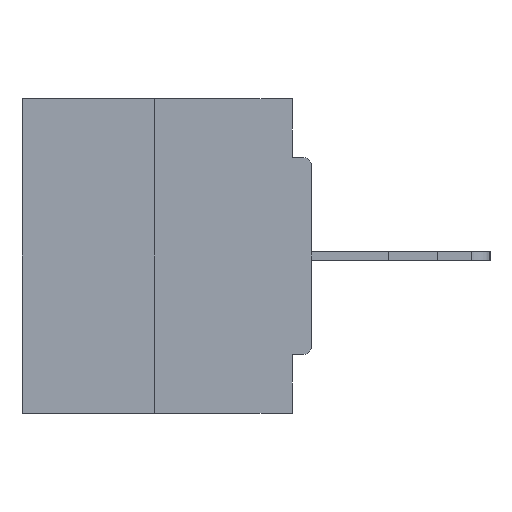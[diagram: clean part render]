
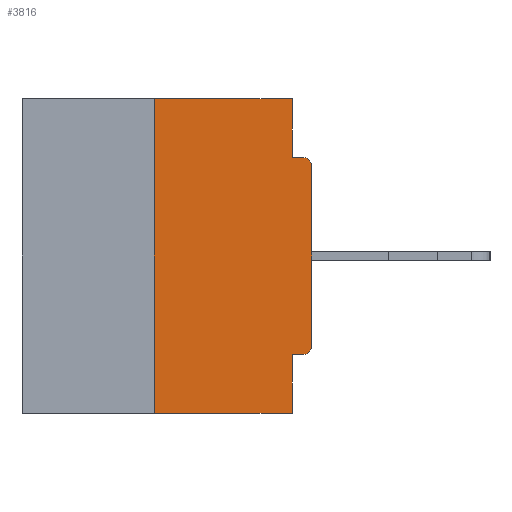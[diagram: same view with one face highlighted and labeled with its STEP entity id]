
A CAD part, left-side view. The second image highlights one B-rep face of the part: STEP entity #3816.
In plain terms, the highlighted planar face has unit normal (-1, 0, 0).
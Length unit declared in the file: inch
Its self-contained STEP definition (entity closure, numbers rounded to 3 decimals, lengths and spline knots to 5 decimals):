
#634 = CIRCLE ( 'NONE', #10946, 0.015 ) ;
#707 = CARTESIAN_POINT ( 'NONE',  ( 0., 0., -0.3915 ) ) ;
#1205 = VECTOR ( 'NONE', #3714, 39.37008 ) ;
#1463 = AXIS2_PLACEMENT_3D ( 'NONE', #26990, #29113, #23156 ) ;
#1750 = CARTESIAN_POINT ( 'NONE',  ( 0., 0., -0.0935 ) ) ;
#2798 = VERTEX_POINT ( 'NONE', #28218 ) ;
#3714 = DIRECTION ( 'NONE',  ( 0., -1., 0. ) ) ;
#3816 = ADVANCED_FACE ( 'NONE', ( #35316 ), #32275, .F. ) ;
#5351 = VERTEX_POINT ( 'NONE', #21413 ) ;
#6648 = VECTOR ( 'NONE', #7829, 39.37008 ) ;
#6746 = LINE ( 'NONE', #18210, #1205 ) ;
#6902 = LINE ( 'NONE', #21577, #28126 ) ;
#7588 = CARTESIAN_POINT ( 'NONE',  ( 0., 0., -0.1085 ) ) ;
#7648 = CARTESIAN_POINT ( 'NONE',  ( 0., 0.031, -0.5 ) ) ;
#7827 = VERTEX_POINT ( 'NONE', #13499 ) ;
#7829 = DIRECTION ( 'NONE',  ( 0., 0., -1. ) ) ;
#8826 = VECTOR ( 'NONE', #36713, 39.37008 ) ;
#8870 = DIRECTION ( 'NONE',  ( 0., 0., -1. ) ) ;
#9846 = EDGE_CURVE ( 'NONE', #5351, #11969, #19815, .T. ) ;
#10120 = EDGE_CURVE ( 'NONE', #11969, #11700, #10551, .T. ) ;
#10477 = DIRECTION ( 'NONE',  ( 0., -1., 0. ) ) ;
#10551 = LINE ( 'NONE', #25041, #8826 ) ;
#10864 = CARTESIAN_POINT ( 'NONE',  ( 0., 0.031, -0.0935 ) ) ;
#10946 = AXIS2_PLACEMENT_3D ( 'NONE', #27232, #33727, #27991 ) ;
#11240 = EDGE_CURVE ( 'NONE', #22677, #28325, #19466, .T. ) ;
#11262 = LINE ( 'NONE', #7648, #6648 ) ;
#11700 = VERTEX_POINT ( 'NONE', #7588 ) ;
#11910 = LINE ( 'NONE', #20702, #14744 ) ;
#11969 = VERTEX_POINT ( 'NONE', #707 ) ;
#12204 = CARTESIAN_POINT ( 'NONE',  ( 0., 0.25, 0. ) ) ;
#12468 = ORIENTED_EDGE ( 'NONE', *, *, #35264, .F. ) ;
#12639 = CARTESIAN_POINT ( 'NONE',  ( 0., 0.015, -0.0935 ) ) ;
#13499 = CARTESIAN_POINT ( 'NONE',  ( 0., 0.25, -0.5 ) ) ;
#14319 = EDGE_CURVE ( 'NONE', #17470, #33353, #11262, .T. ) ;
#14453 = CARTESIAN_POINT ( 'NONE',  ( 0., 0.25, 0. ) ) ;
#14524 = CARTESIAN_POINT ( 'NONE',  ( 0., 0., -0.4065 ) ) ;
#14699 = DIRECTION ( 'NONE',  ( 0., 0., -1. ) ) ;
#14744 = VECTOR ( 'NONE', #8870, 39.37008 ) ;
#15480 = ORIENTED_EDGE ( 'NONE', *, *, #15537, .T. ) ;
#15537 = EDGE_CURVE ( 'NONE', #11700, #28325, #634, .T. ) ;
#17399 = EDGE_CURVE ( 'NONE', #2798, #22677, #11910, .T. ) ;
#17470 = VERTEX_POINT ( 'NONE', #24075 ) ;
#17967 = DIRECTION ( 'NONE',  ( 1., 0., 0. ) ) ;
#17976 = LINE ( 'NONE', #12204, #30230 ) ;
#18210 = CARTESIAN_POINT ( 'NONE',  ( 0., 0.46, -0.5 ) ) ;
#18380 = EDGE_LOOP ( 'NONE', ( #36856, #36719, #27149, #36778, #12468, #18574, #19358, #15480, #20745, #25625 ) ) ;
#18547 = DIRECTION ( 'NONE',  ( 0., -1., 0. ) ) ;
#18574 = ORIENTED_EDGE ( 'NONE', *, *, #9846, .T. ) ;
#19358 = ORIENTED_EDGE ( 'NONE', *, *, #10120, .T. ) ;
#19466 = LINE ( 'NONE', #1750, #28061 ) ;
#19815 = CIRCLE ( 'NONE', #1463, 0.015 ) ;
#20702 = CARTESIAN_POINT ( 'NONE',  ( 0., 0.031, 0. ) ) ;
#20745 = ORIENTED_EDGE ( 'NONE', *, *, #11240, .F. ) ;
#21413 = CARTESIAN_POINT ( 'NONE',  ( 0., 0.015, -0.4065 ) ) ;
#21577 = CARTESIAN_POINT ( 'NONE',  ( 0., 0.46, 0. ) ) ;
#22677 = VERTEX_POINT ( 'NONE', #10864 ) ;
#23156 = DIRECTION ( 'NONE',  ( 0., 0., -1. ) ) ;
#23171 = EDGE_CURVE ( 'NONE', #7827, #30763, #17976, .T. ) ;
#24075 = CARTESIAN_POINT ( 'NONE',  ( 0., 0.031, -0.4065 ) ) ;
#25041 = CARTESIAN_POINT ( 'NONE',  ( 0., 0., 0. ) ) ;
#25625 = ORIENTED_EDGE ( 'NONE', *, *, #17399, .F. ) ;
#26162 = DIRECTION ( 'NONE',  ( 0., 1., 0. ) ) ;
#26534 = CARTESIAN_POINT ( 'NONE',  ( 0., 0.46, 0. ) ) ;
#26990 = CARTESIAN_POINT ( 'NONE',  ( 0., 0.015, -0.3915 ) ) ;
#27097 = EDGE_CURVE ( 'NONE', #7827, #33353, #6746, .T. ) ;
#27149 = ORIENTED_EDGE ( 'NONE', *, *, #27097, .T. ) ;
#27232 = CARTESIAN_POINT ( 'NONE',  ( 0., 0.015, -0.1085 ) ) ;
#27290 = DIRECTION ( 'NONE',  ( 0., 0., 1. ) ) ;
#27991 = DIRECTION ( 'NONE',  ( 0., 0., -1. ) ) ;
#28061 = VECTOR ( 'NONE', #10477, 39.37008 ) ;
#28126 = VECTOR ( 'NONE', #18547, 39.37008 ) ;
#28218 = CARTESIAN_POINT ( 'NONE',  ( 0., 0.031, 0. ) ) ;
#28325 = VERTEX_POINT ( 'NONE', #12639 ) ;
#29042 = AXIS2_PLACEMENT_3D ( 'NONE', #26534, #17967, #14699 ) ;
#29113 = DIRECTION ( 'NONE',  ( -1., 0., 0. ) ) ;
#30041 = EDGE_CURVE ( 'NONE', #30763, #2798, #6902, .T. ) ;
#30230 = VECTOR ( 'NONE', #27290, 39.37008 ) ;
#30763 = VERTEX_POINT ( 'NONE', #14453 ) ;
#30999 = CARTESIAN_POINT ( 'NONE',  ( 0., 0.031, -0.5 ) ) ;
#31914 = LINE ( 'NONE', #14524, #37241 ) ;
#32275 = PLANE ( 'NONE',  #29042 ) ;
#33353 = VERTEX_POINT ( 'NONE', #30999 ) ;
#33727 = DIRECTION ( 'NONE',  ( -1., 0., 0. ) ) ;
#35264 = EDGE_CURVE ( 'NONE', #5351, #17470, #31914, .T. ) ;
#35316 = FACE_OUTER_BOUND ( 'NONE', #18380, .T. ) ;
#36713 = DIRECTION ( 'NONE',  ( 0., 0., 1. ) ) ;
#36719 = ORIENTED_EDGE ( 'NONE', *, *, #23171, .F. ) ;
#36778 = ORIENTED_EDGE ( 'NONE', *, *, #14319, .F. ) ;
#36856 = ORIENTED_EDGE ( 'NONE', *, *, #30041, .F. ) ;
#37241 = VECTOR ( 'NONE', #26162, 39.37008 ) ;
